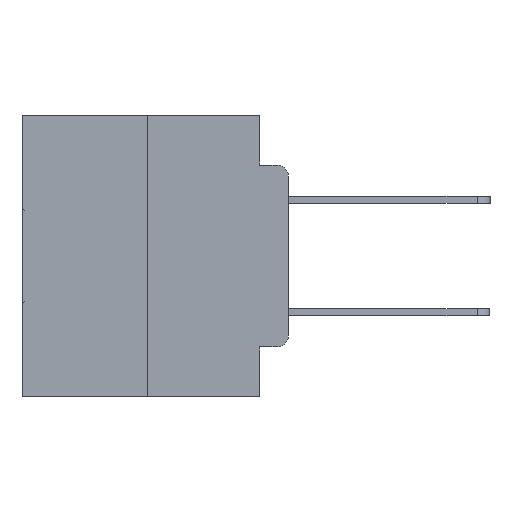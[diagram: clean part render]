
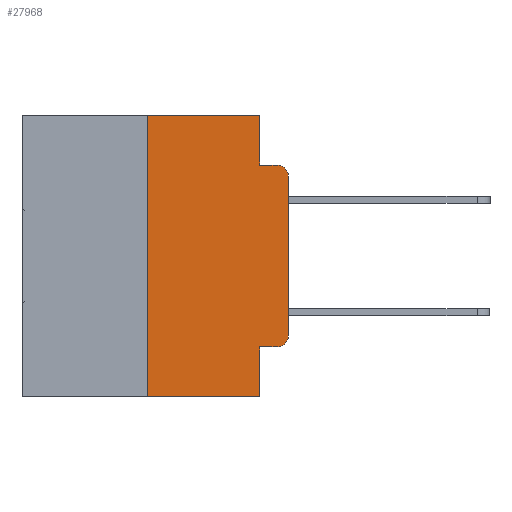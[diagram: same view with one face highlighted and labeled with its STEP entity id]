
A CAD part, left-side view. The second image highlights one B-rep face of the part: STEP entity #27968.
In plain terms, the highlighted planar face has unit normal (-1, 0, 0).
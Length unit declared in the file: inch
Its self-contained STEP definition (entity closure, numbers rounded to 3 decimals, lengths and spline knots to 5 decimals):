
#435 = VERTEX_POINT ( 'NONE', #4848 ) ;
#759 = ORIENTED_EDGE ( 'NONE', *, *, #8649, .F. ) ;
#775 = CARTESIAN_POINT ( 'NONE',  ( 0., 0.051, -0.5 ) ) ;
#946 = VECTOR ( 'NONE', #17108, 39.37008 ) ;
#1087 = CARTESIAN_POINT ( 'NONE',  ( 0., 0., -0.1085 ) ) ;
#1570 = ORIENTED_EDGE ( 'NONE', *, *, #26137, .T. ) ;
#2692 = VECTOR ( 'NONE', #19895, 39.37008 ) ;
#3766 = CARTESIAN_POINT ( 'NONE',  ( 0., 0.02, -0.1085 ) ) ;
#4084 = DIRECTION ( 'NONE',  ( -1., 0., 0. ) ) ;
#4848 = CARTESIAN_POINT ( 'NONE',  ( 0., 0., -0.3915 ) ) ;
#4904 = ORIENTED_EDGE ( 'NONE', *, *, #22173, .T. ) ;
#5505 = CARTESIAN_POINT ( 'NONE',  ( 0., 0.051, -0.4115 ) ) ;
#5623 = LINE ( 'NONE', #5505, #24624 ) ;
#6249 = DIRECTION ( 'NONE',  ( 0., 0., -1. ) ) ;
#6552 = VECTOR ( 'NONE', #8101, 39.37008 ) ;
#7483 = DIRECTION ( 'NONE',  ( 0., -1., 0. ) ) ;
#7997 = DIRECTION ( 'NONE',  ( 0., 0., -1. ) ) ;
#8101 = DIRECTION ( 'NONE',  ( 0., 0., 1. ) ) ;
#8161 = LINE ( 'NONE', #14662, #946 ) ;
#8608 = VERTEX_POINT ( 'NONE', #19692 ) ;
#8649 = EDGE_CURVE ( 'NONE', #9867, #26828, #16493, .T. ) ;
#8913 = VECTOR ( 'NONE', #7483, 39.37008 ) ;
#9442 = EDGE_LOOP ( 'NONE', ( #1570, #15187, #759, #15484, #12073, #15850, #21171, #24662, #4904, #18014 ) ) ;
#9867 = VERTEX_POINT ( 'NONE', #12287 ) ;
#9970 = LINE ( 'NONE', #26238, #15572 ) ;
#10799 = CIRCLE ( 'NONE', #17203, 0.02 ) ;
#12073 = ORIENTED_EDGE ( 'NONE', *, *, #12168, .F. ) ;
#12168 = EDGE_CURVE ( 'NONE', #8608, #25055, #26776, .T. ) ;
#12276 = VERTEX_POINT ( 'NONE', #1087 ) ;
#12287 = CARTESIAN_POINT ( 'NONE',  ( 0., 0.051, -0.0885 ) ) ;
#12619 = AXIS2_PLACEMENT_3D ( 'NONE', #18450, #4084, #20841 ) ;
#12656 = DIRECTION ( 'NONE',  ( 0., -1., 0. ) ) ;
#12790 = CARTESIAN_POINT ( 'NONE',  ( 0., 0.051, 0. ) ) ;
#14049 = VERTEX_POINT ( 'NONE', #15340 ) ;
#14415 = DIRECTION ( 'NONE',  ( 0., 0., -1. ) ) ;
#14662 = CARTESIAN_POINT ( 'NONE',  ( 0., 0.051, 0. ) ) ;
#14745 = AXIS2_PLACEMENT_3D ( 'NONE', #26861, #22275, #7997 ) ;
#14960 = CARTESIAN_POINT ( 'NONE',  ( 0., 0.051, -0.0885 ) ) ;
#14987 = LINE ( 'NONE', #24810, #20617 ) ;
#15187 = ORIENTED_EDGE ( 'NONE', *, *, #16653, .T. ) ;
#15340 = CARTESIAN_POINT ( 'NONE',  ( 0., 0.051, -0.4115 ) ) ;
#15484 = ORIENTED_EDGE ( 'NONE', *, *, #27842, .F. ) ;
#15571 = CARTESIAN_POINT ( 'NONE',  ( 0., 0.25, -0.5 ) ) ;
#15572 = VECTOR ( 'NONE', #14415, 39.37008 ) ;
#15850 = ORIENTED_EDGE ( 'NONE', *, *, #21589, .F. ) ;
#16493 = LINE ( 'NONE', #14960, #2692 ) ;
#16653 = EDGE_CURVE ( 'NONE', #12276, #26828, #10799, .T. ) ;
#17108 = DIRECTION ( 'NONE',  ( 0., 0., -1. ) ) ;
#17203 = AXIS2_PLACEMENT_3D ( 'NONE', #3766, #20554, #6249 ) ;
#17683 = DIRECTION ( 'NONE',  ( 0., 0., 1. ) ) ;
#18014 = ORIENTED_EDGE ( 'NONE', *, *, #20594, .T. ) ;
#18316 = VERTEX_POINT ( 'NONE', #15571 ) ;
#18450 = CARTESIAN_POINT ( 'NONE',  ( 0., 0.02, -0.3915 ) ) ;
#19692 = CARTESIAN_POINT ( 'NONE',  ( 0., 0.25, 0. ) ) ;
#19895 = DIRECTION ( 'NONE',  ( 0., -1., 0. ) ) ;
#19898 = CARTESIAN_POINT ( 'NONE',  ( 0., 0.473, 0. ) ) ;
#19909 = PLANE ( 'NONE',  #14745 ) ;
#20554 = DIRECTION ( 'NONE',  ( -1., 0., 0. ) ) ;
#20594 = EDGE_CURVE ( 'NONE', #23311, #435, #25803, .T. ) ;
#20617 = VECTOR ( 'NONE', #17683, 39.37008 ) ;
#20741 = LINE ( 'NONE', #29282, #6552 ) ;
#20841 = DIRECTION ( 'NONE',  ( 0., 0., -1. ) ) ;
#20851 = LINE ( 'NONE', #24127, #8913 ) ;
#21171 = ORIENTED_EDGE ( 'NONE', *, *, #23647, .T. ) ;
#21589 = EDGE_CURVE ( 'NONE', #18316, #8608, #14987, .T. ) ;
#22116 = DIRECTION ( 'NONE',  ( 0., -1., 0. ) ) ;
#22173 = EDGE_CURVE ( 'NONE', #14049, #23311, #5623, .T. ) ;
#22243 = CARTESIAN_POINT ( 'NONE',  ( 0., 0.02, -0.0885 ) ) ;
#22275 = DIRECTION ( 'NONE',  ( 1., 0., 0. ) ) ;
#23311 = VERTEX_POINT ( 'NONE', #25271 ) ;
#23647 = EDGE_CURVE ( 'NONE', #18316, #26157, #20851, .T. ) ;
#24127 = CARTESIAN_POINT ( 'NONE',  ( 0., 0.473, -0.5 ) ) ;
#24624 = VECTOR ( 'NONE', #22116, 39.37008 ) ;
#24662 = ORIENTED_EDGE ( 'NONE', *, *, #28416, .F. ) ;
#24810 = CARTESIAN_POINT ( 'NONE',  ( 0., 0.25, 0. ) ) ;
#25055 = VERTEX_POINT ( 'NONE', #12790 ) ;
#25271 = CARTESIAN_POINT ( 'NONE',  ( 0., 0.02, -0.4115 ) ) ;
#25803 = CIRCLE ( 'NONE', #12619, 0.02 ) ;
#26071 = VECTOR ( 'NONE', #12656, 39.37008 ) ;
#26137 = EDGE_CURVE ( 'NONE', #435, #12276, #20741, .T. ) ;
#26157 = VERTEX_POINT ( 'NONE', #775 ) ;
#26238 = CARTESIAN_POINT ( 'NONE',  ( 0., 0.051, 0. ) ) ;
#26776 = LINE ( 'NONE', #19898, #26071 ) ;
#26828 = VERTEX_POINT ( 'NONE', #22243 ) ;
#26861 = CARTESIAN_POINT ( 'NONE',  ( 0., 0.473, 0. ) ) ;
#27842 = EDGE_CURVE ( 'NONE', #25055, #9867, #8161, .T. ) ;
#27968 = ADVANCED_FACE ( 'NONE', ( #28163 ), #19909, .F. ) ;
#28163 = FACE_OUTER_BOUND ( 'NONE', #9442, .T. ) ;
#28416 = EDGE_CURVE ( 'NONE', #14049, #26157, #9970, .T. ) ;
#29282 = CARTESIAN_POINT ( 'NONE',  ( 0., 0., 0. ) ) ;
